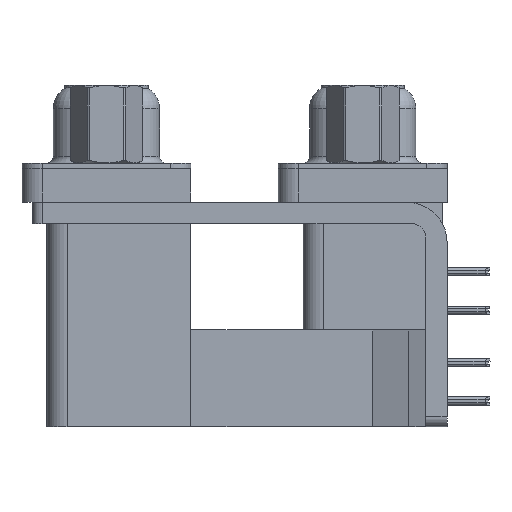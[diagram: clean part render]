
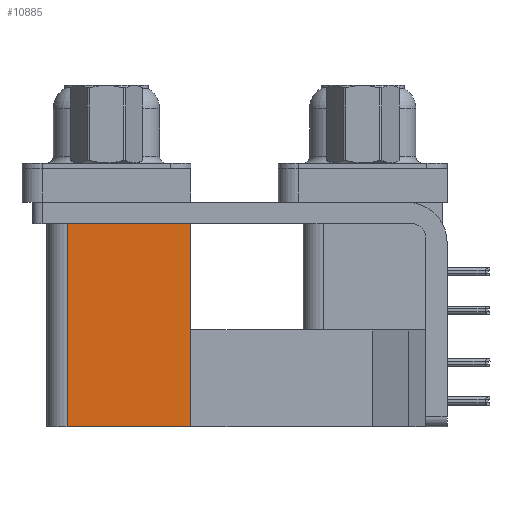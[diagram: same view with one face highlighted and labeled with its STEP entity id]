
A CAD part, left-side view. The second image highlights one B-rep face of the part: STEP entity #10885.
In plain terms, the highlighted planar face has unit normal (-1, 0, 0).
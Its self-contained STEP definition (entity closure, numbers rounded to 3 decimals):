
#1394 = ORIENTED_EDGE ( 'NONE', *, *, #16047, .T. ) ;
#5070 = VECTOR ( 'NONE', #39484, 1000. ) ;
#7930 = CARTESIAN_POINT ( 'NONE',  ( 3.79, 12.775, -19.2 ) ) ;
#8035 = FACE_OUTER_BOUND ( 'NONE', #45742, .T. ) ;
#8424 = ORIENTED_EDGE ( 'NONE', *, *, #11612, .T. ) ;
#8643 = EDGE_CURVE ( 'NONE', #20539, #19627, #28472, .T. ) ;
#10443 = VECTOR ( 'NONE', #38987, 1000. ) ;
#10885 = ADVANCED_FACE ( 'NONE', ( #8035 ), #30008, .F. ) ;
#11612 = EDGE_CURVE ( 'NONE', #30854, #24741, #39007, .T. ) ;
#13130 = EDGE_CURVE ( 'NONE', #30854, #20539, #18807, .T. ) ;
#16047 = EDGE_CURVE ( 'NONE', #24741, #19627, #24750, .T. ) ;
#17695 = CARTESIAN_POINT ( 'NONE',  ( 3.79, 12.775, -2.5 ) ) ;
#18807 = LINE ( 'NONE', #7930, #42770 ) ;
#19627 = VERTEX_POINT ( 'NONE', #33294 ) ;
#20539 = VERTEX_POINT ( 'NONE', #24464 ) ;
#20751 = CARTESIAN_POINT ( 'NONE',  ( 3.79, 12.775, -19.2 ) ) ;
#23634 = VECTOR ( 'NONE', #34473, 1000. ) ;
#24197 = ORIENTED_EDGE ( 'NONE', *, *, #13130, .F. ) ;
#24464 = CARTESIAN_POINT ( 'NONE',  ( 3.79, 21.975, -19.2 ) ) ;
#24741 = VERTEX_POINT ( 'NONE', #26754 ) ;
#24750 = LINE ( 'NONE', #17695, #10443 ) ;
#26680 = DIRECTION ( 'NONE',  ( 0., 1., 0. ) ) ;
#26754 = CARTESIAN_POINT ( 'NONE',  ( 3.79, 12.775, -2.5 ) ) ;
#27091 = AXIS2_PLACEMENT_3D ( 'NONE', #33315, #29778, #26680 ) ;
#28472 = LINE ( 'NONE', #41405, #23634 ) ;
#29778 = DIRECTION ( 'NONE',  ( 1., 0., 0. ) ) ;
#30008 = PLANE ( 'NONE',  #27091 ) ;
#30854 = VERTEX_POINT ( 'NONE', #39307 ) ;
#33294 = CARTESIAN_POINT ( 'NONE',  ( 3.79, 21.975, -2.5 ) ) ;
#33315 = CARTESIAN_POINT ( 'NONE',  ( 3.79, 12.775, -19.2 ) ) ;
#34473 = DIRECTION ( 'NONE',  ( 0., 0., 1. ) ) ;
#38987 = DIRECTION ( 'NONE',  ( 0., 1., 0. ) ) ;
#39007 = LINE ( 'NONE', #20751, #5070 ) ;
#39307 = CARTESIAN_POINT ( 'NONE',  ( 3.79, 12.775, -19.2 ) ) ;
#39484 = DIRECTION ( 'NONE',  ( 0., 0., 1. ) ) ;
#41405 = CARTESIAN_POINT ( 'NONE',  ( 3.79, 21.975, -19.2 ) ) ;
#42770 = VECTOR ( 'NONE', #46822, 1000. ) ;
#44039 = ORIENTED_EDGE ( 'NONE', *, *, #8643, .F. ) ;
#45742 = EDGE_LOOP ( 'NONE', ( #1394, #44039, #24197, #8424 ) ) ;
#46822 = DIRECTION ( 'NONE',  ( 0., 1., 0. ) ) ;
